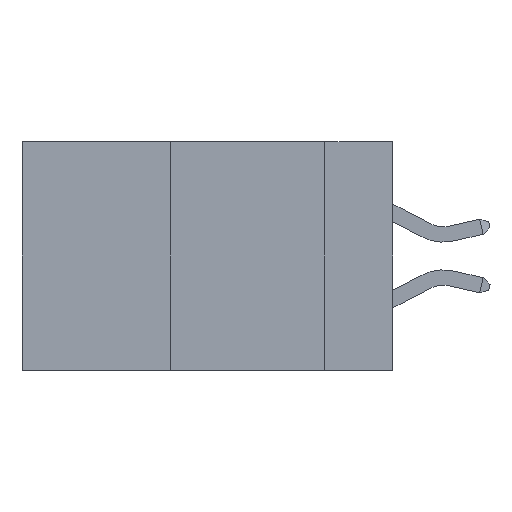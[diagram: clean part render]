
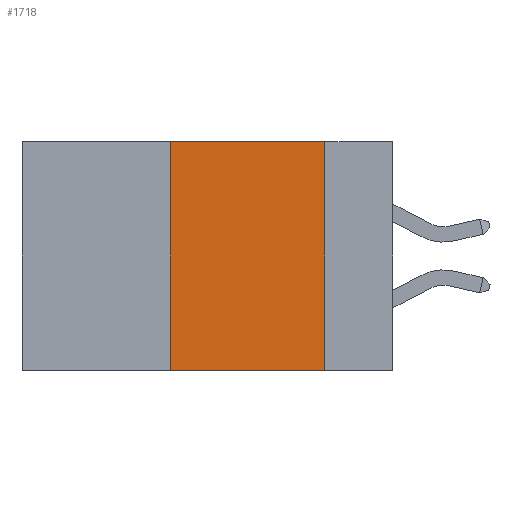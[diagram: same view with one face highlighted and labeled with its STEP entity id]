
A CAD part, left-side view. The second image highlights one B-rep face of the part: STEP entity #1718.
In plain terms, the highlighted planar face has unit normal (-1, 0, 0).
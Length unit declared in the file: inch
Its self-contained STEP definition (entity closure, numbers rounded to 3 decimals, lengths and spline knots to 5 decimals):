
#1718 = ADVANCED_FACE ( 'NONE', ( #23226 ), #12866, .F. ) ;
#2253 = VERTEX_POINT ( 'NONE', #14715 ) ;
#2305 = DIRECTION ( 'NONE',  ( 1., 0., 0. ) ) ;
#2603 = VECTOR ( 'NONE', #30988, 39.37008 ) ;
#5499 = VECTOR ( 'NONE', #14149, 39.37008 ) ;
#5935 = DIRECTION ( 'NONE',  ( 0., -1., 0. ) ) ;
#6320 = VECTOR ( 'NONE', #17623, 39.37008 ) ;
#6548 = VERTEX_POINT ( 'NONE', #24587 ) ;
#10509 = ORIENTED_EDGE ( 'NONE', *, *, #18956, .F. ) ;
#10617 = EDGE_CURVE ( 'NONE', #6548, #16914, #12796, .T. ) ;
#10918 = ORIENTED_EDGE ( 'NONE', *, *, #10617, .T. ) ;
#11236 = EDGE_CURVE ( 'NONE', #6548, #24002, #21326, .T. ) ;
#12329 = ORIENTED_EDGE ( 'NONE', *, *, #11236, .F. ) ;
#12796 = LINE ( 'NONE', #25402, #2603 ) ;
#12866 = PLANE ( 'NONE',  #32138 ) ;
#13431 = EDGE_CURVE ( 'NONE', #24002, #2253, #24606, .T. ) ;
#14149 = DIRECTION ( 'NONE',  ( 0., 0., 1. ) ) ;
#14715 = CARTESIAN_POINT ( 'NONE',  ( 0., 0.11, 0. ) ) ;
#15217 = VECTOR ( 'NONE', #5935, 39.37008 ) ;
#16914 = VERTEX_POINT ( 'NONE', #17787 ) ;
#17623 = DIRECTION ( 'NONE',  ( 0., 0., -1. ) ) ;
#17787 = CARTESIAN_POINT ( 'NONE',  ( 0., 0.11, -0.37 ) ) ;
#18247 = DIRECTION ( 'NONE',  ( 0., 0., -1. ) ) ;
#18602 = CARTESIAN_POINT ( 'NONE',  ( 0., 0.6, 0. ) ) ;
#18956 = EDGE_CURVE ( 'NONE', #2253, #16914, #33660, .T. ) ;
#19450 = CARTESIAN_POINT ( 'NONE',  ( 0., 0.36, 0. ) ) ;
#21326 = LINE ( 'NONE', #19450, #5499 ) ;
#22890 = CARTESIAN_POINT ( 'NONE',  ( 0., 0.11, 0. ) ) ;
#23226 = FACE_OUTER_BOUND ( 'NONE', #27732, .T. ) ;
#24002 = VERTEX_POINT ( 'NONE', #32795 ) ;
#24587 = CARTESIAN_POINT ( 'NONE',  ( 0., 0.36, -0.37 ) ) ;
#24606 = LINE ( 'NONE', #30668, #15217 ) ;
#25402 = CARTESIAN_POINT ( 'NONE',  ( 0., 0.6, -0.37 ) ) ;
#27732 = EDGE_LOOP ( 'NONE', ( #10509, #32377, #12329, #10918 ) ) ;
#30668 = CARTESIAN_POINT ( 'NONE',  ( 0., 0.6, 0. ) ) ;
#30988 = DIRECTION ( 'NONE',  ( 0., -1., 0. ) ) ;
#32138 = AXIS2_PLACEMENT_3D ( 'NONE', #18602, #2305, #18247 ) ;
#32377 = ORIENTED_EDGE ( 'NONE', *, *, #13431, .F. ) ;
#32795 = CARTESIAN_POINT ( 'NONE',  ( 0., 0.36, 0. ) ) ;
#33660 = LINE ( 'NONE', #22890, #6320 ) ;
